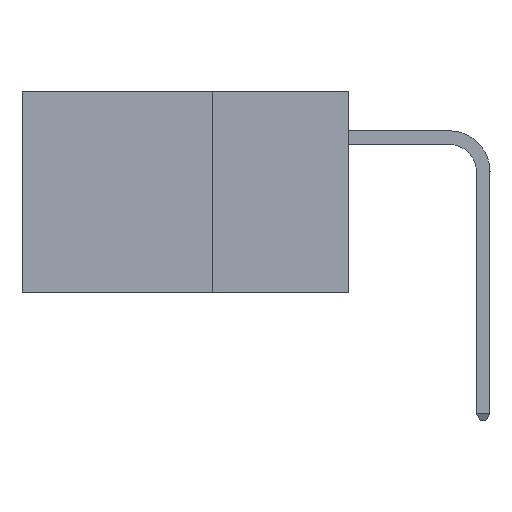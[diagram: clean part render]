
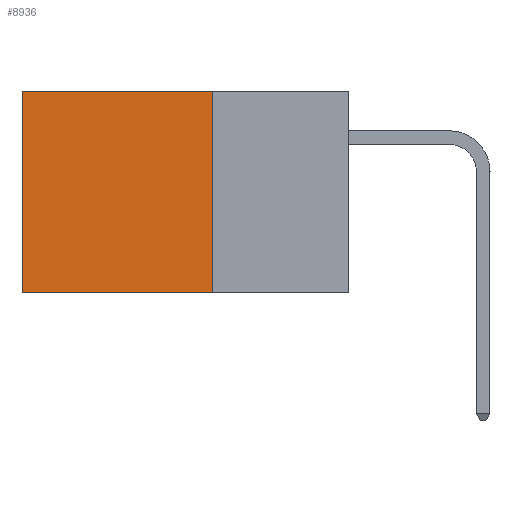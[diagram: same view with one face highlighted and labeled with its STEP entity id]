
A CAD part, left-side view. The second image highlights one B-rep face of the part: STEP entity #8936.
In plain terms, the highlighted planar face has unit normal (-1, 0, 0).
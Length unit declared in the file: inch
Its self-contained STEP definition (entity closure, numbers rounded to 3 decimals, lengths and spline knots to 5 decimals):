
#571 = CARTESIAN_POINT ( 'NONE',  ( 0.2875, 0.25, -0.37 ) ) ;
#774 = EDGE_CURVE ( 'NONE', #18167, #11452, #24960, .T. ) ;
#1076 = PLANE ( 'NONE',  #36460 ) ;
#3462 = CARTESIAN_POINT ( 'NONE',  ( 0.2875, 0.6, 0. ) ) ;
#4379 = DIRECTION ( 'NONE',  ( 0., 0., -1. ) ) ;
#5478 = CARTESIAN_POINT ( 'NONE',  ( 0.2875, 0.25, 0. ) ) ;
#7930 = VECTOR ( 'NONE', #26309, 39.37008 ) ;
#8154 = CARTESIAN_POINT ( 'NONE',  ( 0.2875, 0.25, -0.37 ) ) ;
#8936 = ADVANCED_FACE ( 'NONE', ( #39066 ), #1076, .F. ) ;
#9374 = VERTEX_POINT ( 'NONE', #3462 ) ;
#10072 = VERTEX_POINT ( 'NONE', #10217 ) ;
#10217 = CARTESIAN_POINT ( 'NONE',  ( 0.2875, 0.6, -0.37 ) ) ;
#10368 = CARTESIAN_POINT ( 'NONE',  ( 0.2875, 0.25, 0. ) ) ;
#11452 = VERTEX_POINT ( 'NONE', #8154 ) ;
#11761 = DIRECTION ( 'NONE',  ( 0., 1., 0. ) ) ;
#15129 = EDGE_CURVE ( 'NONE', #11452, #10072, #25556, .T. ) ;
#15242 = VECTOR ( 'NONE', #11761, 39.37008 ) ;
#16105 = VECTOR ( 'NONE', #23103, 39.37008 ) ;
#17761 = ORIENTED_EDGE ( 'NONE', *, *, #15129, .F. ) ;
#18167 = VERTEX_POINT ( 'NONE', #5478 ) ;
#20444 = CARTESIAN_POINT ( 'NONE',  ( 0.2875, 0.25, 0. ) ) ;
#20456 = LINE ( 'NONE', #39052, #27853 ) ;
#21555 = ORIENTED_EDGE ( 'NONE', *, *, #38293, .T. ) ;
#23103 = DIRECTION ( 'NONE',  ( 0., 1., 0. ) ) ;
#23367 = DIRECTION ( 'NONE',  ( 0., 0., -1. ) ) ;
#23615 = DIRECTION ( 'NONE',  ( 1., 0., 0. ) ) ;
#24960 = LINE ( 'NONE', #10368, #7930 ) ;
#25556 = LINE ( 'NONE', #571, #16105 ) ;
#26309 = DIRECTION ( 'NONE',  ( 0., 0., -1. ) ) ;
#27240 = EDGE_LOOP ( 'NONE', ( #21555, #17761, #36559, #29163 ) ) ;
#27621 = CARTESIAN_POINT ( 'NONE',  ( 0.2875, 0.25, 0. ) ) ;
#27853 = VECTOR ( 'NONE', #23367, 39.37008 ) ;
#29163 = ORIENTED_EDGE ( 'NONE', *, *, #40445, .T. ) ;
#32052 = LINE ( 'NONE', #27621, #15242 ) ;
#36460 = AXIS2_PLACEMENT_3D ( 'NONE', #20444, #23615, #4379 ) ;
#36559 = ORIENTED_EDGE ( 'NONE', *, *, #774, .F. ) ;
#38293 = EDGE_CURVE ( 'NONE', #9374, #10072, #20456, .T. ) ;
#39052 = CARTESIAN_POINT ( 'NONE',  ( 0.2875, 0.6, 0. ) ) ;
#39066 = FACE_OUTER_BOUND ( 'NONE', #27240, .T. ) ;
#40445 = EDGE_CURVE ( 'NONE', #18167, #9374, #32052, .T. ) ;
